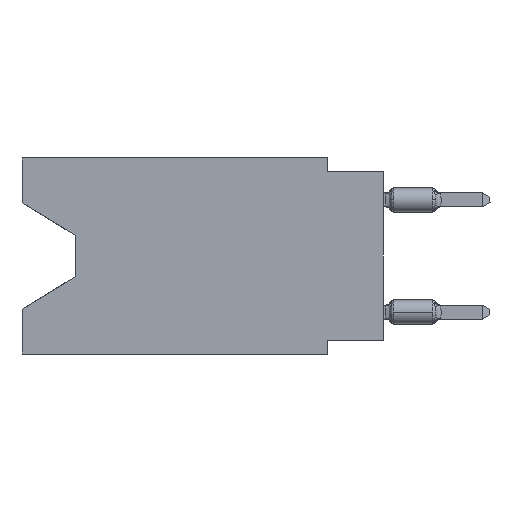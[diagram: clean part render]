
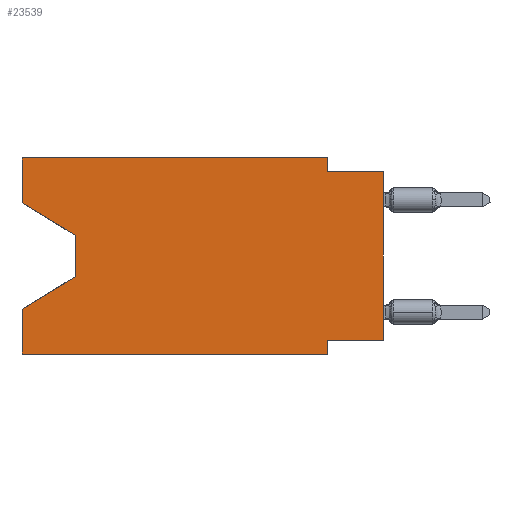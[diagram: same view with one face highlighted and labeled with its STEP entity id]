
A CAD part, left-side view. The second image highlights one B-rep face of the part: STEP entity #23539.
In plain terms, the highlighted planar face has unit normal (-1, 0, 0).
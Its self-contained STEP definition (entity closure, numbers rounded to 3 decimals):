
#150 = VECTOR ( 'NONE', #12544, 1000. ) ;
#337 = LINE ( 'NONE', #36743, #150 ) ;
#1133 = LINE ( 'NONE', #25152, #22874 ) ;
#1404 = EDGE_LOOP ( 'NONE', ( #23862, #10391, #26119, #21017, #33181, #24402, #16572, #21388, #32725, #5078, #10847, #16962 ) ) ;
#1636 = CARTESIAN_POINT ( 'NONE',  ( 0., 13.97, -3.505 ) ) ;
#1755 = VERTEX_POINT ( 'NONE', #31720 ) ;
#2478 = EDGE_CURVE ( 'NONE', #6702, #2950, #19554, .T. ) ;
#2950 = VERTEX_POINT ( 'NONE', #26578 ) ;
#3433 = LINE ( 'NONE', #28020, #14501 ) ;
#3975 = LINE ( 'NONE', #15782, #15222 ) ;
#4070 = VECTOR ( 'NONE', #4218, 1000. ) ;
#4218 = DIRECTION ( 'NONE',  ( 0., -1., 0. ) ) ;
#4486 = DIRECTION ( 'NONE',  ( 0., 1., 0. ) ) ;
#4900 = CARTESIAN_POINT ( 'NONE',  ( 0., 16.383, 0. ) ) ;
#5078 = ORIENTED_EDGE ( 'NONE', *, *, #36843, .F. ) ;
#5881 = EDGE_CURVE ( 'NONE', #25031, #36121, #25550, .T. ) ;
#6291 = VECTOR ( 'NONE', #36927, 1000. ) ;
#6702 = VERTEX_POINT ( 'NONE', #20142 ) ;
#7146 = VECTOR ( 'NONE', #22595, 1000. ) ;
#7278 = DIRECTION ( 'NONE',  ( 1., 0., 0. ) ) ;
#7517 = VERTEX_POINT ( 'NONE', #11844 ) ;
#7812 = LINE ( 'NONE', #31818, #37869 ) ;
#8820 = LINE ( 'NONE', #20625, #33800 ) ;
#9005 = EDGE_CURVE ( 'NONE', #1755, #14153, #25261, .T. ) ;
#9746 = CARTESIAN_POINT ( 'NONE',  ( 0., 2.54, -8.89 ) ) ;
#10272 = EDGE_CURVE ( 'NONE', #7517, #31132, #1133, .T. ) ;
#10391 = ORIENTED_EDGE ( 'NONE', *, *, #9005, .T. ) ;
#10847 = ORIENTED_EDGE ( 'NONE', *, *, #36984, .F. ) ;
#11680 = CARTESIAN_POINT ( 'NONE',  ( 0., 16.383, -6.852 ) ) ;
#11844 = CARTESIAN_POINT ( 'NONE',  ( 0., 0., -8.255 ) ) ;
#12117 = VERTEX_POINT ( 'NONE', #35033 ) ;
#12544 = DIRECTION ( 'NONE',  ( 0., 0., -1. ) ) ;
#12664 = DIRECTION ( 'NONE',  ( 0., -1., 0. ) ) ;
#13265 = LINE ( 'NONE', #25058, #17522 ) ;
#14023 = EDGE_CURVE ( 'NONE', #12117, #24489, #13265, .T. ) ;
#14153 = VERTEX_POINT ( 'NONE', #26228 ) ;
#14501 = VECTOR ( 'NONE', #15437, 1000. ) ;
#15043 = CARTESIAN_POINT ( 'NONE',  ( 0., 2.54, -8.89 ) ) ;
#15222 = VECTOR ( 'NONE', #32585, 1000. ) ;
#15237 = LINE ( 'NONE', #15043, #23257 ) ;
#15437 = DIRECTION ( 'NONE',  ( 0., 0., 1. ) ) ;
#15782 = CARTESIAN_POINT ( 'NONE',  ( 0., 16.383, -2.038 ) ) ;
#15883 = DIRECTION ( 'NONE',  ( 0., -1., 0. ) ) ;
#16572 = ORIENTED_EDGE ( 'NONE', *, *, #10272, .F. ) ;
#16962 = ORIENTED_EDGE ( 'NONE', *, *, #5881, .F. ) ;
#17522 = VECTOR ( 'NONE', #12664, 1000. ) ;
#18193 = CARTESIAN_POINT ( 'NONE',  ( 0., 16.383, 0. ) ) ;
#19265 = DIRECTION ( 'NONE',  ( 0., 0., -1. ) ) ;
#19554 = LINE ( 'NONE', #31185, #4070 ) ;
#20142 = CARTESIAN_POINT ( 'NONE',  ( 0., 2.54, -0.635 ) ) ;
#20625 = CARTESIAN_POINT ( 'NONE',  ( 0., 16.383, 0. ) ) ;
#20815 = DIRECTION ( 'NONE',  ( 0., 0., 1. ) ) ;
#21017 = ORIENTED_EDGE ( 'NONE', *, *, #21797, .F. ) ;
#21388 = ORIENTED_EDGE ( 'NONE', *, *, #32605, .T. ) ;
#21797 = EDGE_CURVE ( 'NONE', #12117, #36508, #8820, .T. ) ;
#22595 = DIRECTION ( 'NONE',  ( 0., 0., 1. ) ) ;
#22874 = VECTOR ( 'NONE', #4486, 1000. ) ;
#23257 = VECTOR ( 'NONE', #27040, 1000. ) ;
#23539 = ADVANCED_FACE ( 'NONE', ( #38163 ), #37581, .F. ) ;
#23862 = ORIENTED_EDGE ( 'NONE', *, *, #34754, .T. ) ;
#24402 = ORIENTED_EDGE ( 'NONE', *, *, #29474, .F. ) ;
#24489 = VERTEX_POINT ( 'NONE', #9746 ) ;
#25031 = VERTEX_POINT ( 'NONE', #29944 ) ;
#25058 = CARTESIAN_POINT ( 'NONE',  ( 0., 16.383, -8.89 ) ) ;
#25152 = CARTESIAN_POINT ( 'NONE',  ( 0., 0., -8.255 ) ) ;
#25261 = LINE ( 'NONE', #1636, #27892 ) ;
#25550 = LINE ( 'NONE', #37560, #7146 ) ;
#26119 = ORIENTED_EDGE ( 'NONE', *, *, #32131, .T. ) ;
#26228 = CARTESIAN_POINT ( 'NONE',  ( 0., 13.97, -5.385 ) ) ;
#26578 = CARTESIAN_POINT ( 'NONE',  ( 0., 0., -0.635 ) ) ;
#27040 = DIRECTION ( 'NONE',  ( 0., 0., -1. ) ) ;
#27778 = VERTEX_POINT ( 'NONE', #29055 ) ;
#27892 = VECTOR ( 'NONE', #28605, 1000. ) ;
#28020 = CARTESIAN_POINT ( 'NONE',  ( 0., 0., 0. ) ) ;
#28605 = DIRECTION ( 'NONE',  ( 0., 0., -1. ) ) ;
#29055 = CARTESIAN_POINT ( 'NONE',  ( 0., 2.54, 0. ) ) ;
#29474 = EDGE_CURVE ( 'NONE', #31132, #24489, #15237, .T. ) ;
#29944 = CARTESIAN_POINT ( 'NONE',  ( 0., 16.383, -2.038 ) ) ;
#30830 = CARTESIAN_POINT ( 'NONE',  ( 0., 13.97, -5.385 ) ) ;
#31132 = VERTEX_POINT ( 'NONE', #38819 ) ;
#31185 = CARTESIAN_POINT ( 'NONE',  ( 0., 0., -0.635 ) ) ;
#31720 = CARTESIAN_POINT ( 'NONE',  ( 0., 13.97, -3.505 ) ) ;
#31818 = CARTESIAN_POINT ( 'NONE',  ( 0., 16.383, 0. ) ) ;
#32131 = EDGE_CURVE ( 'NONE', #14153, #36508, #34367, .T. ) ;
#32585 = DIRECTION ( 'NONE',  ( 0., -0.855, -0.519 ) ) ;
#32605 = EDGE_CURVE ( 'NONE', #7517, #2950, #3433, .T. ) ;
#32725 = ORIENTED_EDGE ( 'NONE', *, *, #2478, .F. ) ;
#33181 = ORIENTED_EDGE ( 'NONE', *, *, #14023, .T. ) ;
#33800 = VECTOR ( 'NONE', #20815, 1000. ) ;
#34367 = LINE ( 'NONE', #30830, #6291 ) ;
#34754 = EDGE_CURVE ( 'NONE', #25031, #1755, #3975, .T. ) ;
#35033 = CARTESIAN_POINT ( 'NONE',  ( 0., 16.383, -8.89 ) ) ;
#36121 = VERTEX_POINT ( 'NONE', #18193 ) ;
#36508 = VERTEX_POINT ( 'NONE', #11680 ) ;
#36743 = CARTESIAN_POINT ( 'NONE',  ( 0., 2.54, 0. ) ) ;
#36843 = EDGE_CURVE ( 'NONE', #27778, #6702, #337, .T. ) ;
#36927 = DIRECTION ( 'NONE',  ( 0., 0.855, -0.519 ) ) ;
#36984 = EDGE_CURVE ( 'NONE', #36121, #27778, #7812, .T. ) ;
#37560 = CARTESIAN_POINT ( 'NONE',  ( 0., 16.383, 0. ) ) ;
#37581 = PLANE ( 'NONE',  #38052 ) ;
#37869 = VECTOR ( 'NONE', #15883, 1000. ) ;
#38052 = AXIS2_PLACEMENT_3D ( 'NONE', #4900, #7278, #19265 ) ;
#38163 = FACE_OUTER_BOUND ( 'NONE', #1404, .T. ) ;
#38819 = CARTESIAN_POINT ( 'NONE',  ( 0., 2.54, -8.255 ) ) ;
